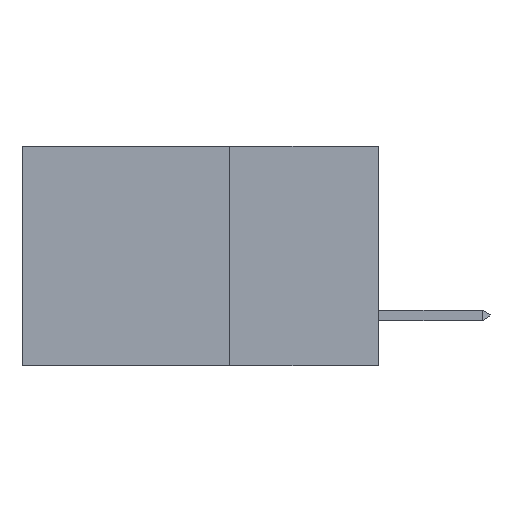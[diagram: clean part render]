
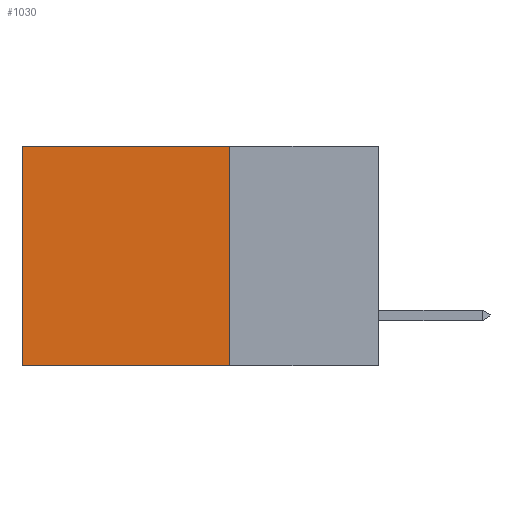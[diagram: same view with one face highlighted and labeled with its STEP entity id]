
A CAD part, left-side view. The second image highlights one B-rep face of the part: STEP entity #1030.
In plain terms, the highlighted planar face has unit normal (-1, 0, 0).
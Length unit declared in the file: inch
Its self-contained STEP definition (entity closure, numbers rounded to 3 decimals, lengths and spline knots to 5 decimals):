
#112 = EDGE_LOOP ( 'NONE', ( #10400, #5837, #3835, #12340 ) ) ;
#504 = LINE ( 'NONE', #4822, #994 ) ;
#548 = LINE ( 'NONE', #4865, #6222 ) ;
#598 = VECTOR ( 'NONE', #10290, 39.37008 ) ;
#793 = CARTESIAN_POINT ( 'NONE',  ( 0.2615, 0.6, -0.37 ) ) ;
#994 = VECTOR ( 'NONE', #3838, 39.37008 ) ;
#1030 = ADVANCED_FACE ( 'NONE', ( #9186 ), #12585, .F. ) ;
#1220 = VECTOR ( 'NONE', #2648, 39.37008 ) ;
#1517 = LINE ( 'NONE', #9085, #1220 ) ;
#1575 = CARTESIAN_POINT ( 'NONE',  ( 0.2615, 0.25, -0.37 ) ) ;
#1981 = EDGE_CURVE ( 'NONE', #9896, #5609, #504, .T. ) ;
#2096 = CARTESIAN_POINT ( 'NONE',  ( 0.2615, 0.6, -0.37 ) ) ;
#2340 = AXIS2_PLACEMENT_3D ( 'NONE', #2740, #13562, #7061 ) ;
#2648 = DIRECTION ( 'NONE',  ( 0., 1., 0. ) ) ;
#2740 = CARTESIAN_POINT ( 'NONE',  ( 0.2615, 0.25, -0.37 ) ) ;
#3835 = ORIENTED_EDGE ( 'NONE', *, *, #10199, .F. ) ;
#3838 = DIRECTION ( 'NONE',  ( 0., 1., 0. ) ) ;
#4564 = EDGE_CURVE ( 'NONE', #5120, #5609, #12624, .T. ) ;
#4822 = CARTESIAN_POINT ( 'NONE',  ( 0.2615, 0.25, -0.37 ) ) ;
#4865 = CARTESIAN_POINT ( 'NONE',  ( 0.2615, 0.25, -0.37 ) ) ;
#5120 = VERTEX_POINT ( 'NONE', #10878 ) ;
#5524 = DIRECTION ( 'NONE',  ( 0., 0., -1. ) ) ;
#5609 = VERTEX_POINT ( 'NONE', #2096 ) ;
#5837 = ORIENTED_EDGE ( 'NONE', *, *, #1981, .F. ) ;
#6222 = VECTOR ( 'NONE', #5524, 39.37008 ) ;
#7061 = DIRECTION ( 'NONE',  ( 0., 0., -1. ) ) ;
#7700 = CARTESIAN_POINT ( 'NONE',  ( 0.2615, 0.25, 0. ) ) ;
#8732 = EDGE_CURVE ( 'NONE', #10394, #5120, #1517, .T. ) ;
#9085 = CARTESIAN_POINT ( 'NONE',  ( 0.2615, 0.25, 0. ) ) ;
#9186 = FACE_OUTER_BOUND ( 'NONE', #112, .T. ) ;
#9896 = VERTEX_POINT ( 'NONE', #1575 ) ;
#10199 = EDGE_CURVE ( 'NONE', #10394, #9896, #548, .T. ) ;
#10290 = DIRECTION ( 'NONE',  ( 0., 0., -1. ) ) ;
#10394 = VERTEX_POINT ( 'NONE', #7700 ) ;
#10400 = ORIENTED_EDGE ( 'NONE', *, *, #4564, .T. ) ;
#10878 = CARTESIAN_POINT ( 'NONE',  ( 0.2615, 0.6, 0. ) ) ;
#12340 = ORIENTED_EDGE ( 'NONE', *, *, #8732, .T. ) ;
#12585 = PLANE ( 'NONE',  #2340 ) ;
#12624 = LINE ( 'NONE', #793, #598 ) ;
#13562 = DIRECTION ( 'NONE',  ( 1., 0., 0. ) ) ;
